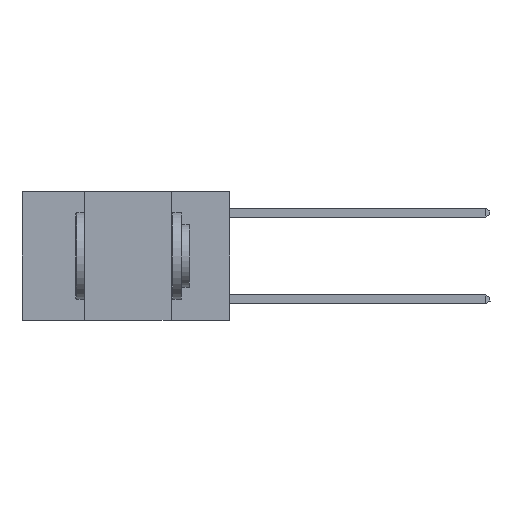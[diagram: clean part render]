
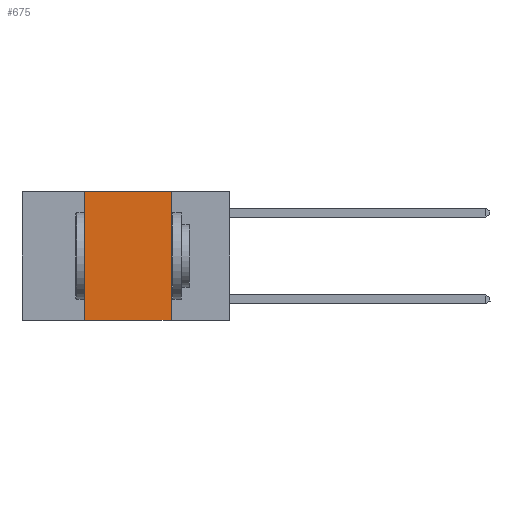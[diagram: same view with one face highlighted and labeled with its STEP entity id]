
A CAD part, left-side view. The second image highlights one B-rep face of the part: STEP entity #675.
In plain terms, the highlighted planar face has unit normal (-1, 0, 0).
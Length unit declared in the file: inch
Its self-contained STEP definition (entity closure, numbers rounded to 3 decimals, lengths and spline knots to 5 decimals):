
#4 = CARTESIAN_POINT ( 'NONE',  ( 0., 0.42, 0. ) ) ;
#675 = ADVANCED_FACE ( 'NONE', ( #17645 ), #3255, .F. ) ;
#1950 = AXIS2_PLACEMENT_3D ( 'NONE', #13065, #5281, #19080 ) ;
#3076 = ORIENTED_EDGE ( 'NONE', *, *, #23895, .F. ) ;
#3255 = PLANE ( 'NONE',  #1950 ) ;
#3985 = VERTEX_POINT ( 'NONE', #4 ) ;
#4075 = VECTOR ( 'NONE', #10376, 39.37008 ) ;
#4132 = VERTEX_POINT ( 'NONE', #21165 ) ;
#4691 = LINE ( 'NONE', #8400, #4075 ) ;
#4959 = EDGE_CURVE ( 'NONE', #10084, #3985, #14710, .T. ) ;
#5281 = DIRECTION ( 'NONE',  ( 1., 0., 0. ) ) ;
#8400 = CARTESIAN_POINT ( 'NONE',  ( 0., 0.17, 0. ) ) ;
#9460 = VECTOR ( 'NONE', #11719, 39.37008 ) ;
#9663 = CARTESIAN_POINT ( 'NONE',  ( 0., 0.42, 0. ) ) ;
#10084 = VERTEX_POINT ( 'NONE', #11860 ) ;
#10376 = DIRECTION ( 'NONE',  ( 0., 0., -1. ) ) ;
#10441 = LINE ( 'NONE', #12929, #15682 ) ;
#10791 = ORIENTED_EDGE ( 'NONE', *, *, #19842, .F. ) ;
#10885 = DIRECTION ( 'NONE',  ( 0., -1., 0. ) ) ;
#11719 = DIRECTION ( 'NONE',  ( 0., 0., 1. ) ) ;
#11860 = CARTESIAN_POINT ( 'NONE',  ( 0., 0.42, -0.37 ) ) ;
#12814 = VECTOR ( 'NONE', #10885, 39.37008 ) ;
#12882 = ORIENTED_EDGE ( 'NONE', *, *, #17061, .T. ) ;
#12929 = CARTESIAN_POINT ( 'NONE',  ( 0., 0.6, -0.37 ) ) ;
#13065 = CARTESIAN_POINT ( 'NONE',  ( 0., 0.6, 0. ) ) ;
#13439 = LINE ( 'NONE', #22705, #12814 ) ;
#14710 = LINE ( 'NONE', #9663, #9460 ) ;
#15682 = VECTOR ( 'NONE', #18788, 39.37008 ) ;
#17061 = EDGE_CURVE ( 'NONE', #10084, #22299, #10441, .T. ) ;
#17645 = FACE_OUTER_BOUND ( 'NONE', #17969, .T. ) ;
#17969 = EDGE_LOOP ( 'NONE', ( #10791, #3076, #24761, #12882 ) ) ;
#18788 = DIRECTION ( 'NONE',  ( 0., -1., 0. ) ) ;
#19080 = DIRECTION ( 'NONE',  ( 0., 0., -1. ) ) ;
#19842 = EDGE_CURVE ( 'NONE', #4132, #22299, #4691, .T. ) ;
#21165 = CARTESIAN_POINT ( 'NONE',  ( 0., 0.17, 0. ) ) ;
#21899 = CARTESIAN_POINT ( 'NONE',  ( 0., 0.17, -0.37 ) ) ;
#22299 = VERTEX_POINT ( 'NONE', #21899 ) ;
#22705 = CARTESIAN_POINT ( 'NONE',  ( 0., 0.6, 0. ) ) ;
#23895 = EDGE_CURVE ( 'NONE', #3985, #4132, #13439, .T. ) ;
#24761 = ORIENTED_EDGE ( 'NONE', *, *, #4959, .F. ) ;
